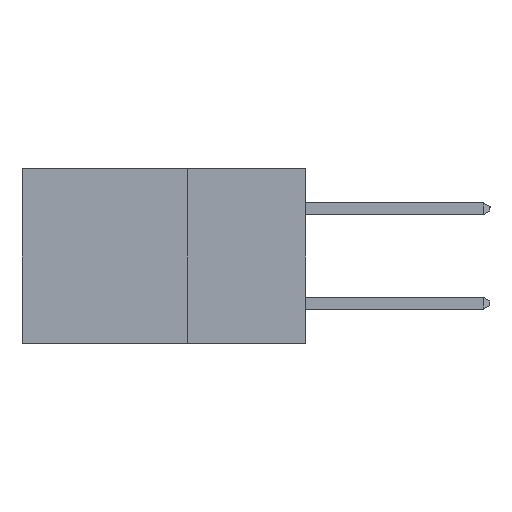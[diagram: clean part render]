
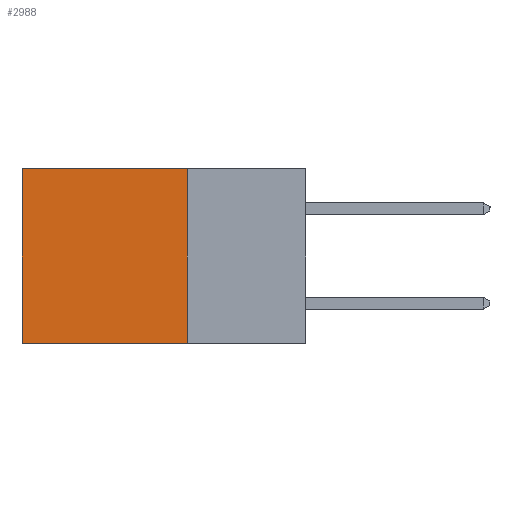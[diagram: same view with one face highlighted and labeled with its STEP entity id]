
A CAD part, left-side view. The second image highlights one B-rep face of the part: STEP entity #2988.
In plain terms, the highlighted planar face has unit normal (-1, 0, 0).
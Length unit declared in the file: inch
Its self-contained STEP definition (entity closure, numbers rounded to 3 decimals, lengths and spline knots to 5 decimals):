
#517 = VERTEX_POINT ( 'NONE', #2697 ) ;
#770 = DIRECTION ( 'NONE',  ( 1., 0., 0. ) ) ;
#822 = PLANE ( 'NONE',  #2931 ) ;
#1162 = VERTEX_POINT ( 'NONE', #1555 ) ;
#1194 = ORIENTED_EDGE ( 'NONE', *, *, #4483, .F. ) ;
#1555 = CARTESIAN_POINT ( 'NONE',  ( 0.2615, 0.6, -0.37 ) ) ;
#1696 = VECTOR ( 'NONE', #4052, 39.37008 ) ;
#1835 = LINE ( 'NONE', #5579, #3690 ) ;
#2287 = CARTESIAN_POINT ( 'NONE',  ( 0.2615, 0.6, -0.37 ) ) ;
#2424 = ORIENTED_EDGE ( 'NONE', *, *, #3461, .F. ) ;
#2449 = ORIENTED_EDGE ( 'NONE', *, *, #8829, .T. ) ;
#2697 = CARTESIAN_POINT ( 'NONE',  ( 0.2615, 0.25, -0.37 ) ) ;
#2889 = DIRECTION ( 'NONE',  ( 0., 1., 0. ) ) ;
#2931 = AXIS2_PLACEMENT_3D ( 'NONE', #5208, #770, #8161 ) ;
#2941 = LINE ( 'NONE', #2287, #9046 ) ;
#2988 = ADVANCED_FACE ( 'NONE', ( #5306 ), #822, .F. ) ;
#3461 = EDGE_CURVE ( 'NONE', #517, #1162, #1835, .T. ) ;
#3690 = VECTOR ( 'NONE', #7653, 39.37008 ) ;
#4001 = CARTESIAN_POINT ( 'NONE',  ( 0.2615, 0.25, -0.37 ) ) ;
#4052 = DIRECTION ( 'NONE',  ( 0., 0., -1. ) ) ;
#4109 = CARTESIAN_POINT ( 'NONE',  ( 0.2615, 0.25, 0. ) ) ;
#4483 = EDGE_CURVE ( 'NONE', #6442, #517, #4726, .T. ) ;
#4726 = LINE ( 'NONE', #4001, #1696 ) ;
#5208 = CARTESIAN_POINT ( 'NONE',  ( 0.2615, 0.25, -0.37 ) ) ;
#5306 = FACE_OUTER_BOUND ( 'NONE', #8690, .T. ) ;
#5579 = CARTESIAN_POINT ( 'NONE',  ( 0.2615, 0.25, -0.37 ) ) ;
#5762 = EDGE_CURVE ( 'NONE', #6442, #6633, #7277, .T. ) ;
#6442 = VERTEX_POINT ( 'NONE', #6646 ) ;
#6633 = VERTEX_POINT ( 'NONE', #8762 ) ;
#6646 = CARTESIAN_POINT ( 'NONE',  ( 0.2615, 0.25, 0. ) ) ;
#7277 = LINE ( 'NONE', #4109, #7894 ) ;
#7333 = DIRECTION ( 'NONE',  ( 0., 0., -1. ) ) ;
#7653 = DIRECTION ( 'NONE',  ( 0., 1., 0. ) ) ;
#7894 = VECTOR ( 'NONE', #2889, 39.37008 ) ;
#8161 = DIRECTION ( 'NONE',  ( 0., 0., -1. ) ) ;
#8525 = ORIENTED_EDGE ( 'NONE', *, *, #5762, .T. ) ;
#8690 = EDGE_LOOP ( 'NONE', ( #2449, #2424, #1194, #8525 ) ) ;
#8762 = CARTESIAN_POINT ( 'NONE',  ( 0.2615, 0.6, 0. ) ) ;
#8829 = EDGE_CURVE ( 'NONE', #6633, #1162, #2941, .T. ) ;
#9046 = VECTOR ( 'NONE', #7333, 39.37008 ) ;
